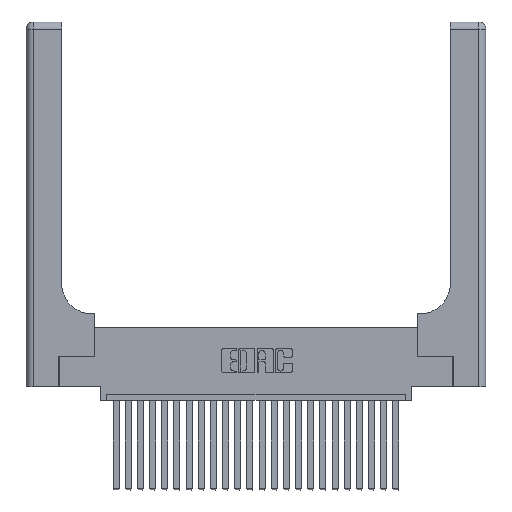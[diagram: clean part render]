
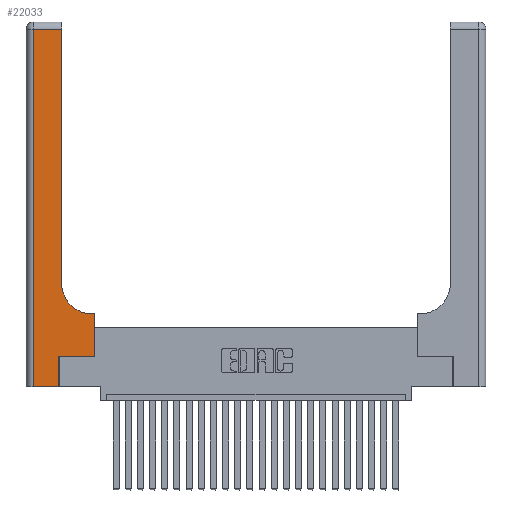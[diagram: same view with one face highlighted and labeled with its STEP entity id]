
A CAD part, top view. The second image highlights one B-rep face of the part: STEP entity #22033.
In plain terms, the highlighted planar face has unit normal (0, 0, 1).
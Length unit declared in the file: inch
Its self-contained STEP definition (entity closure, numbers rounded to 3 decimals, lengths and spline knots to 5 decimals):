
#849 = EDGE_CURVE ( 'NONE', #6387, #23887, #11077, .T. ) ;
#922 = VECTOR ( 'NONE', #18779, 39.37008 ) ;
#1867 = EDGE_CURVE ( 'NONE', #19370, #6737, #18654, .T. ) ;
#1921 = ORIENTED_EDGE ( 'NONE', *, *, #849, .T. ) ;
#2193 = VECTOR ( 'NONE', #21938, 39.37008 ) ;
#2212 = CARTESIAN_POINT ( 'NONE',  ( 0.269, 0., 0.37 ) ) ;
#2473 = FACE_OUTER_BOUND ( 'NONE', #4083, .T. ) ;
#2569 = VERTEX_POINT ( 'NONE', #3154 ) ;
#2819 = VERTEX_POINT ( 'NONE', #21696 ) ;
#2928 = LINE ( 'NONE', #3850, #12775 ) ;
#3154 = CARTESIAN_POINT ( 'NONE',  ( 0.5585, 0.6, 0.37 ) ) ;
#3460 = DIRECTION ( 'NONE',  ( 0., 1., 0. ) ) ;
#3850 = CARTESIAN_POINT ( 'NONE',  ( 0.2915, 3., 0.37 ) ) ;
#4040 = EDGE_CURVE ( 'NONE', #15401, #2819, #12706, .T. ) ;
#4055 = VECTOR ( 'NONE', #3460, 39.37008 ) ;
#4083 = EDGE_LOOP ( 'NONE', ( #7315, #24015, #17802, #25389, #17379, #1921, #6438, #13811, #9679 ) ) ;
#4375 = CARTESIAN_POINT ( 'NONE',  ( 0.2915, 2.94, 0.37 ) ) ;
#4893 = EDGE_CURVE ( 'NONE', #2569, #15401, #8081, .T. ) ;
#6387 = VERTEX_POINT ( 'NONE', #6423 ) ;
#6423 = CARTESIAN_POINT ( 'NONE',  ( 0.269, 0.25, 0.37 ) ) ;
#6433 = DIRECTION ( 'NONE',  ( 1., 0., 0. ) ) ;
#6438 = ORIENTED_EDGE ( 'NONE', *, *, #9493, .T. ) ;
#6737 = VERTEX_POINT ( 'NONE', #9950 ) ;
#7315 = ORIENTED_EDGE ( 'NONE', *, *, #12482, .T. ) ;
#7324 = EDGE_CURVE ( 'NONE', #7566, #19370, #8559, .T. ) ;
#7566 = VERTEX_POINT ( 'NONE', #4375 ) ;
#7611 = CARTESIAN_POINT ( 'NONE',  ( 0.269, 0., 0.37 ) ) ;
#7632 = CARTESIAN_POINT ( 'NONE',  ( 0.269, 0.25, 0.37 ) ) ;
#7966 = EDGE_CURVE ( 'NONE', #13975, #6387, #9654, .T. ) ;
#8048 = CARTESIAN_POINT ( 'NONE',  ( 0., 3., 0.37 ) ) ;
#8081 = LINE ( 'NONE', #15836, #21299 ) ;
#8559 = LINE ( 'NONE', #23837, #22724 ) ;
#8805 = CARTESIAN_POINT ( 'NONE',  ( 0., 0., 0.37 ) ) ;
#9123 = CARTESIAN_POINT ( 'NONE',  ( 0.06, 3., 0.37 ) ) ;
#9208 = DIRECTION ( 'NONE',  ( 0., -1., 0. ) ) ;
#9493 = EDGE_CURVE ( 'NONE', #23887, #2569, #15119, .T. ) ;
#9654 = LINE ( 'NONE', #2212, #2193 ) ;
#9657 = DIRECTION ( 'NONE',  ( 0., 1., 0. ) ) ;
#9679 = ORIENTED_EDGE ( 'NONE', *, *, #4040, .T. ) ;
#9950 = CARTESIAN_POINT ( 'NONE',  ( 0.06, 0., 0.37 ) ) ;
#11060 = AXIS2_PLACEMENT_3D ( 'NONE', #24556, #24382, #6433 ) ;
#11077 = LINE ( 'NONE', #7632, #19076 ) ;
#11749 = CARTESIAN_POINT ( 'NONE',  ( 0.5585, 0.25, 0.37 ) ) ;
#12176 = DIRECTION ( 'NONE',  ( -1., 0., 0. ) ) ;
#12395 = CARTESIAN_POINT ( 'NONE',  ( 0.5585, 0.25, 0.37 ) ) ;
#12482 = EDGE_CURVE ( 'NONE', #2819, #7566, #2928, .T. ) ;
#12706 = CIRCLE ( 'NONE', #11060, 0.25 ) ;
#12775 = VECTOR ( 'NONE', #9657, 39.37008 ) ;
#13018 = AXIS2_PLACEMENT_3D ( 'NONE', #8048, #17865, #14024 ) ;
#13811 = ORIENTED_EDGE ( 'NONE', *, *, #4893, .T. ) ;
#13869 = PLANE ( 'NONE',  #13018 ) ;
#13975 = VERTEX_POINT ( 'NONE', #7611 ) ;
#14024 = DIRECTION ( 'NONE',  ( -1., 0., 0. ) ) ;
#15119 = LINE ( 'NONE', #11749, #4055 ) ;
#15401 = VERTEX_POINT ( 'NONE', #23926 ) ;
#15836 = CARTESIAN_POINT ( 'NONE',  ( 0.2915, 0.6, 0.37 ) ) ;
#17347 = DIRECTION ( 'NONE',  ( 1., 0., 0. ) ) ;
#17379 = ORIENTED_EDGE ( 'NONE', *, *, #7966, .T. ) ;
#17802 = ORIENTED_EDGE ( 'NONE', *, *, #1867, .T. ) ;
#17865 = DIRECTION ( 'NONE',  ( 0., 0., -1. ) ) ;
#18654 = LINE ( 'NONE', #9123, #22346 ) ;
#18779 = DIRECTION ( 'NONE',  ( 1., 0., 0. ) ) ;
#19076 = VECTOR ( 'NONE', #17347, 39.37008 ) ;
#19370 = VERTEX_POINT ( 'NONE', #24763 ) ;
#19806 = DIRECTION ( 'NONE',  ( -1., 0., 0. ) ) ;
#21299 = VECTOR ( 'NONE', #19806, 39.37008 ) ;
#21696 = CARTESIAN_POINT ( 'NONE',  ( 0.2915, 0.85, 0.37 ) ) ;
#21938 = DIRECTION ( 'NONE',  ( 0., 1., 0. ) ) ;
#22033 = ADVANCED_FACE ( 'NONE', ( #2473 ), #13869, .F. ) ;
#22346 = VECTOR ( 'NONE', #9208, 39.37008 ) ;
#22362 = EDGE_CURVE ( 'NONE', #6737, #13975, #23451, .T. ) ;
#22724 = VECTOR ( 'NONE', #12176, 39.37008 ) ;
#23451 = LINE ( 'NONE', #8805, #922 ) ;
#23837 = CARTESIAN_POINT ( 'NONE',  ( 0., 2.94, 0.37 ) ) ;
#23887 = VERTEX_POINT ( 'NONE', #12395 ) ;
#23926 = CARTESIAN_POINT ( 'NONE',  ( 0.5415, 0.6, 0.37 ) ) ;
#24015 = ORIENTED_EDGE ( 'NONE', *, *, #7324, .T. ) ;
#24382 = DIRECTION ( 'NONE',  ( 0., 0., -1. ) ) ;
#24556 = CARTESIAN_POINT ( 'NONE',  ( 0.5415, 0.85, 0.37 ) ) ;
#24763 = CARTESIAN_POINT ( 'NONE',  ( 0.06, 2.94, 0.37 ) ) ;
#25389 = ORIENTED_EDGE ( 'NONE', *, *, #22362, .T. ) ;
